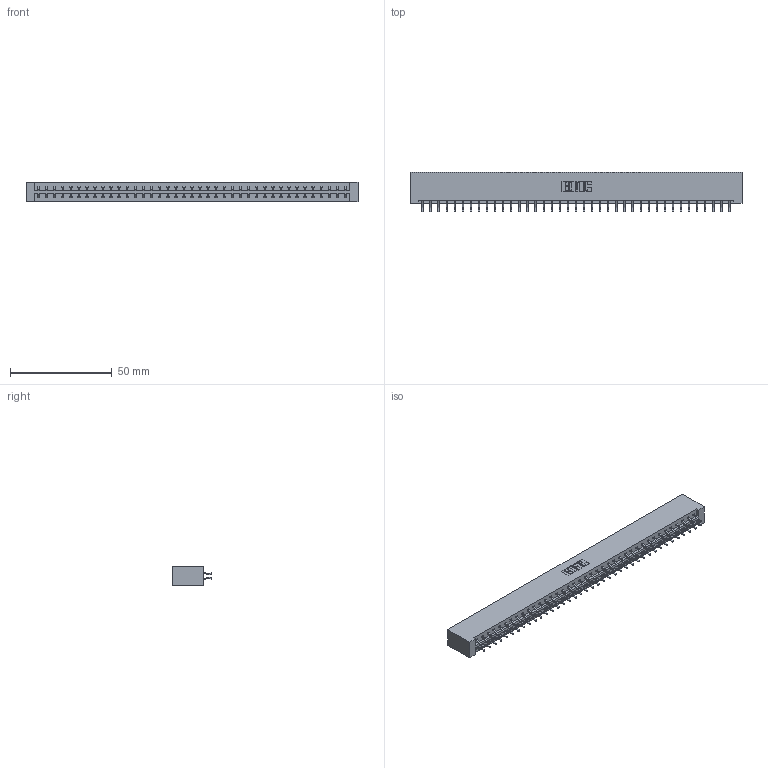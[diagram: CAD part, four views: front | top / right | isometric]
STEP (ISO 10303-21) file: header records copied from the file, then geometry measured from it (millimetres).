
FILE_DESCRIPTION (( 'STEP AP203' ), '1' );
FILE_NAME ('833-078-556-201.STEP', '2020-06-05T20:34:45', ( '' ), ( '' ), 'SwSTEP 2.0', 'SolidWorks 2020', '' );
FILE_SCHEMA (( 'CONFIG_CONTROL_DESIGN' ));
Length unit declared in the file: inch
Products named in the file (3): 833-078-556-201; 345-292-001_556 Tail; 833 Part_Lugless
Assembly tree (79 placements, depth 2):
  833-078-556-201
    833 Part_Lugless
    345-292-001_556 Tail  x78
Bounding box: 162.79 x 19.57 x 9.4 mm (x, y, z)
Volume: 17220.9 mm3; surface area: 20274.5 mm2
Topology: 79 solids, 79 shells, 4630 faces, 13781 edges, 9082 vertices
Faces by surface type: plane 3186, cylinder 1444
Entity records: 25421 total; most frequent: CARTESIAN_POINT 4230, ORIENTED_EDGE 4154, DIRECTION 3601, EDGE_CURVE 2077, VECTOR 1949, LINE 1949, VERTEX_POINT 1382, AXIS2_PLACEMENT_3D 826
